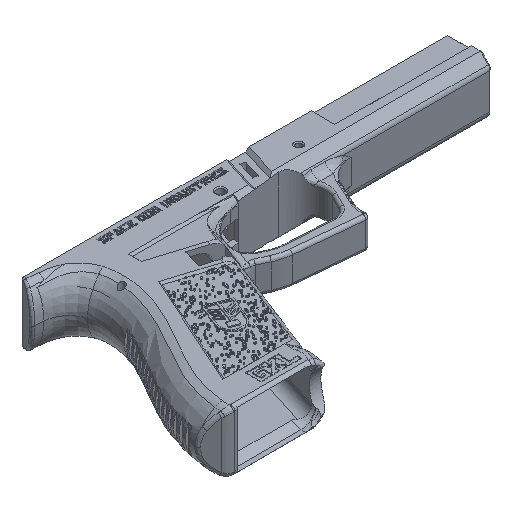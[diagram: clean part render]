
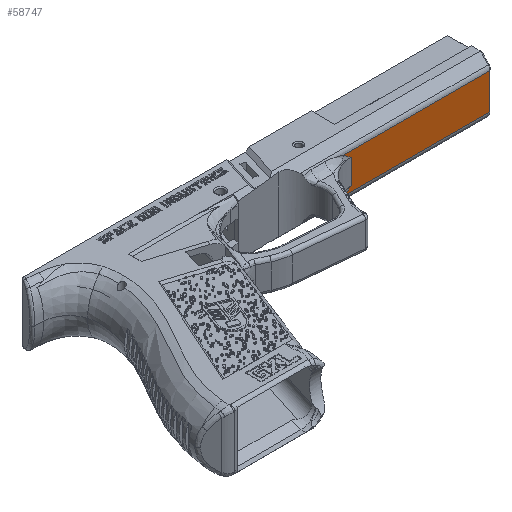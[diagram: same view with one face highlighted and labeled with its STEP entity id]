
A CAD part, isometric view. The second image highlights one B-rep face of the part: STEP entity #58747.
In plain terms, the highlighted planar face has unit normal (0, -1, 0).
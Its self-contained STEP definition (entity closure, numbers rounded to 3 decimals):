
#6434=B_SPLINE_CURVE_WITH_KNOTS('',3,(#70506,#70507,#70508,#70509,#70510,
#70511),.UNSPECIFIED.,.F.,.F.,(4,2,4),(-1.495,-1.493,
-1.066),.UNSPECIFIED.);
#6435=B_SPLINE_CURVE_WITH_KNOTS('',3,(#70514,#70515,#70516,#70517,#70518,
#70519),.UNSPECIFIED.,.F.,.F.,(4,2,4),(-0.427,0.,0.001),
 .UNSPECIFIED.);
#8370=FACE_OUTER_BOUND('',#11926,.T.);
#11926=EDGE_LOOP('',(#39148,#39149,#39150,#39151,#39152,#39153));
#15937=LINE('',#70424,#19788);
#15959=LINE('',#70474,#19810);
#15960=LINE('',#70504,#19811);
#15961=LINE('',#70513,#19812);
#19788=VECTOR('',#63764,10.);
#19810=VECTOR('',#63812,3.);
#19811=VECTOR('',#63815,3.);
#19812=VECTOR('',#63816,10.);
#23633=VERTEX_POINT('',#70417);
#23635=VERTEX_POINT('',#70422);
#23650=VERTEX_POINT('',#70473);
#23654=VERTEX_POINT('',#70503);
#23655=VERTEX_POINT('',#70505);
#23656=VERTEX_POINT('',#70512);
#29796=EDGE_CURVE('',#23635,#23633,#15937,.T.);
#29822=EDGE_CURVE('',#23633,#23650,#15959,.T.);
#29827=EDGE_CURVE('',#23654,#23635,#15960,.T.);
#29828=EDGE_CURVE('',#23655,#23654,#6434,.T.);
#29829=EDGE_CURVE('',#23656,#23655,#15961,.T.);
#29830=EDGE_CURVE('',#23650,#23656,#6435,.T.);
#39148=ORIENTED_EDGE('',*,*,#29796,.F.);
#39149=ORIENTED_EDGE('',*,*,#29827,.F.);
#39150=ORIENTED_EDGE('',*,*,#29828,.F.);
#39151=ORIENTED_EDGE('',*,*,#29829,.F.);
#39152=ORIENTED_EDGE('',*,*,#29830,.F.);
#39153=ORIENTED_EDGE('',*,*,#29822,.F.);
#57647=PLANE('',#62325);
#58747=ADVANCED_FACE('',(#8370),#57647,.F.);
#62325=AXIS2_PLACEMENT_3D('',#70502,#63813,#63814);
#63764=DIRECTION('',(0.,0.,-1.));
#63812=DIRECTION('',(-1.,0.,0.));
#63813=DIRECTION('center_axis',(0.,1.,0.));
#63814=DIRECTION('ref_axis',(0.,0.,
1.));
#63815=DIRECTION('',(1.,0.,0.));
#63816=DIRECTION('',(0.,0.,1.));
#70417=CARTESIAN_POINT('',(178.635,-18.787,19.906));
#70422=CARTESIAN_POINT('',(178.635,-18.787,37.153));
#70424=CARTESIAN_POINT('',(178.635,-18.787,28.529));
#70473=CARTESIAN_POINT('',(107.968,-18.787,19.906));
#70474=CARTESIAN_POINT('',(82.772,-18.787,19.906));
#70502=CARTESIAN_POINT('Origin',(75.926,-18.787,28.529));
#70503=CARTESIAN_POINT('',(107.968,-18.787,37.153));
#70504=CARTESIAN_POINT('',(50.545,-18.787,37.153));
#70505=CARTESIAN_POINT('',(111.379,-18.787,34.49));
#70506=CARTESIAN_POINT('Ctrl Pts',(111.379,-18.787,34.49));
#70507=CARTESIAN_POINT('Ctrl Pts',(111.375,-18.787,34.493));
#70508=CARTESIAN_POINT('Ctrl Pts',(111.372,-18.787,34.496));
#70509=CARTESIAN_POINT('Ctrl Pts',(110.26,-18.787,35.395));
#70510=CARTESIAN_POINT('Ctrl Pts',(109.135,-18.787,36.306));
#70511=CARTESIAN_POINT('Ctrl Pts',(107.968,-18.787,37.153));
#70512=CARTESIAN_POINT('',(111.379,-18.787,22.568));
#70513=CARTESIAN_POINT('',(111.379,-18.787,24.774));
#70514=CARTESIAN_POINT('Ctrl Pts',(107.968,-18.787,19.906));
#70515=CARTESIAN_POINT('Ctrl Pts',(109.135,-18.787,20.752));
#70516=CARTESIAN_POINT('Ctrl Pts',(110.26,-18.787,21.663));
#70517=CARTESIAN_POINT('Ctrl Pts',(111.372,-18.787,22.563));
#70518=CARTESIAN_POINT('Ctrl Pts',(111.375,-18.787,22.566));
#70519=CARTESIAN_POINT('Ctrl Pts',(111.379,-18.787,22.568));
